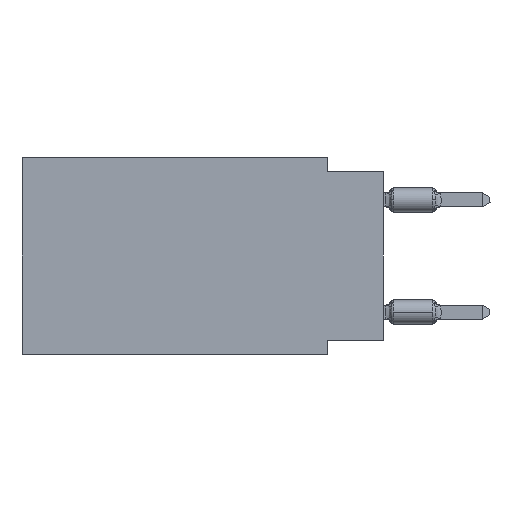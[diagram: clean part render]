
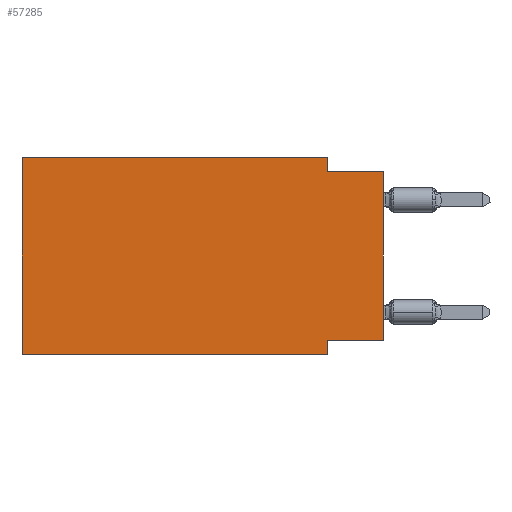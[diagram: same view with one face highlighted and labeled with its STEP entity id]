
A CAD part, left-side view. The second image highlights one B-rep face of the part: STEP entity #57285.
In plain terms, the highlighted planar face has unit normal (-1, 0, 0).
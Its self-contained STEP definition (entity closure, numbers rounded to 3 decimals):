
#1583 = DIRECTION ( 'NONE',  ( 1., 0., 0. ) ) ;
#1924 = VERTEX_POINT ( 'NONE', #14031 ) ;
#1988 = CARTESIAN_POINT ( 'NONE',  ( 0., 16.383, 0. ) ) ;
#2228 = EDGE_LOOP ( 'NONE', ( #8141, #41091, #49540, #36773, #13152, #38510, #17490, #6178 ) ) ;
#2835 = CARTESIAN_POINT ( 'NONE',  ( 0., 16.383, 0. ) ) ;
#4056 = VECTOR ( 'NONE', #34486, 1000. ) ;
#5022 = LINE ( 'NONE', #23142, #11211 ) ;
#5386 = PLANE ( 'NONE',  #51473 ) ;
#5409 = DIRECTION ( 'NONE',  ( 0., 0., 1. ) ) ;
#6178 = ORIENTED_EDGE ( 'NONE', *, *, #15192, .F. ) ;
#7276 = VECTOR ( 'NONE', #55556, 1000. ) ;
#8141 = ORIENTED_EDGE ( 'NONE', *, *, #35946, .T. ) ;
#9043 = VECTOR ( 'NONE', #41319, 1000. ) ;
#10015 = LINE ( 'NONE', #23469, #9043 ) ;
#10018 = VERTEX_POINT ( 'NONE', #53950 ) ;
#10388 = CARTESIAN_POINT ( 'NONE',  ( 0., 16.383, 0. ) ) ;
#10586 = EDGE_CURVE ( 'NONE', #54328, #29846, #37680, .T. ) ;
#11211 = VECTOR ( 'NONE', #28112, 1000. ) ;
#12628 = CARTESIAN_POINT ( 'NONE',  ( 0., 2.54, -0.635 ) ) ;
#13152 = ORIENTED_EDGE ( 'NONE', *, *, #31346, .F. ) ;
#13977 = VERTEX_POINT ( 'NONE', #12628 ) ;
#14031 = CARTESIAN_POINT ( 'NONE',  ( 0., 0., -0.635 ) ) ;
#15192 = EDGE_CURVE ( 'NONE', #44892, #54328, #51651, .T. ) ;
#15937 = CARTESIAN_POINT ( 'NONE',  ( 0., 0., -8.255 ) ) ;
#16555 = EDGE_CURVE ( 'NONE', #44476, #49372, #24488, .T. ) ;
#17490 = ORIENTED_EDGE ( 'NONE', *, *, #10586, .F. ) ;
#18408 = EDGE_CURVE ( 'NONE', #10018, #29846, #46611, .T. ) ;
#18833 = CARTESIAN_POINT ( 'NONE',  ( 0., 16.383, 0. ) ) ;
#23142 = CARTESIAN_POINT ( 'NONE',  ( 0., 2.54, 0. ) ) ;
#23469 = CARTESIAN_POINT ( 'NONE',  ( 0., 0., 0. ) ) ;
#23792 = VECTOR ( 'NONE', #28310, 1000. ) ;
#24488 = LINE ( 'NONE', #1988, #23792 ) ;
#28112 = DIRECTION ( 'NONE',  ( 0., 0., -1. ) ) ;
#28310 = DIRECTION ( 'NONE',  ( 0., -1., 0. ) ) ;
#28793 = LINE ( 'NONE', #10388, #53521 ) ;
#29846 = VERTEX_POINT ( 'NONE', #57153 ) ;
#31346 = EDGE_CURVE ( 'NONE', #10018, #44476, #28793, .T. ) ;
#31376 = VECTOR ( 'NONE', #55394, 1000. ) ;
#34486 = DIRECTION ( 'NONE',  ( 0., -1., 0. ) ) ;
#35946 = EDGE_CURVE ( 'NONE', #44892, #1924, #10015, .T. ) ;
#36089 = CARTESIAN_POINT ( 'NONE',  ( 0., 2.54, 0. ) ) ;
#36773 = ORIENTED_EDGE ( 'NONE', *, *, #16555, .F. ) ;
#37680 = LINE ( 'NONE', #50874, #7276 ) ;
#38510 = ORIENTED_EDGE ( 'NONE', *, *, #18408, .T. ) ;
#38598 = CARTESIAN_POINT ( 'NONE',  ( 0., 0., -0.635 ) ) ;
#41091 = ORIENTED_EDGE ( 'NONE', *, *, #45926, .F. ) ;
#41297 = VECTOR ( 'NONE', #52232, 1000. ) ;
#41319 = DIRECTION ( 'NONE',  ( 0., 0., 1. ) ) ;
#44476 = VERTEX_POINT ( 'NONE', #2835 ) ;
#44892 = VERTEX_POINT ( 'NONE', #46899 ) ;
#44900 = DIRECTION ( 'NONE',  ( 0., 0., -1. ) ) ;
#45771 = FACE_OUTER_BOUND ( 'NONE', #2228, .T. ) ;
#45926 = EDGE_CURVE ( 'NONE', #13977, #1924, #47101, .T. ) ;
#46314 = CARTESIAN_POINT ( 'NONE',  ( 0., 16.383, -8.89 ) ) ;
#46611 = LINE ( 'NONE', #46314, #31376 ) ;
#46899 = CARTESIAN_POINT ( 'NONE',  ( 0., 0., -8.255 ) ) ;
#47101 = LINE ( 'NONE', #38598, #4056 ) ;
#48672 = EDGE_CURVE ( 'NONE', #49372, #13977, #5022, .T. ) ;
#49372 = VERTEX_POINT ( 'NONE', #36089 ) ;
#49540 = ORIENTED_EDGE ( 'NONE', *, *, #48672, .F. ) ;
#50874 = CARTESIAN_POINT ( 'NONE',  ( 0., 2.54, -8.89 ) ) ;
#51473 = AXIS2_PLACEMENT_3D ( 'NONE', #18833, #1583, #44900 ) ;
#51651 = LINE ( 'NONE', #15937, #41297 ) ;
#52232 = DIRECTION ( 'NONE',  ( 0., 1., 0. ) ) ;
#52909 = CARTESIAN_POINT ( 'NONE',  ( 0., 2.54, -8.255 ) ) ;
#53521 = VECTOR ( 'NONE', #5409, 1000. ) ;
#53950 = CARTESIAN_POINT ( 'NONE',  ( 0., 16.383, -8.89 ) ) ;
#54328 = VERTEX_POINT ( 'NONE', #52909 ) ;
#55394 = DIRECTION ( 'NONE',  ( 0., -1., 0. ) ) ;
#55556 = DIRECTION ( 'NONE',  ( 0., 0., -1. ) ) ;
#57153 = CARTESIAN_POINT ( 'NONE',  ( 0., 2.54, -8.89 ) ) ;
#57285 = ADVANCED_FACE ( 'NONE', ( #45771 ), #5386, .F. ) ;
